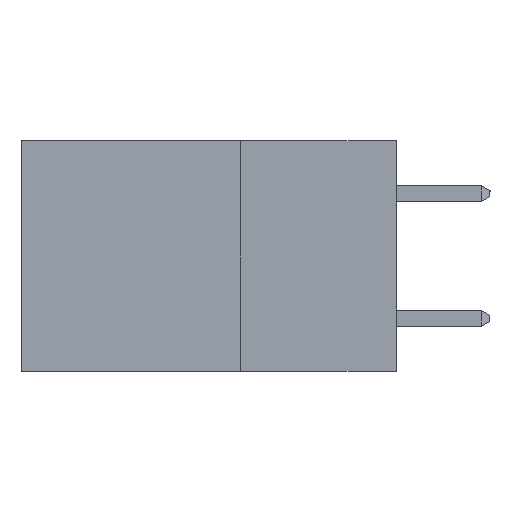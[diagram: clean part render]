
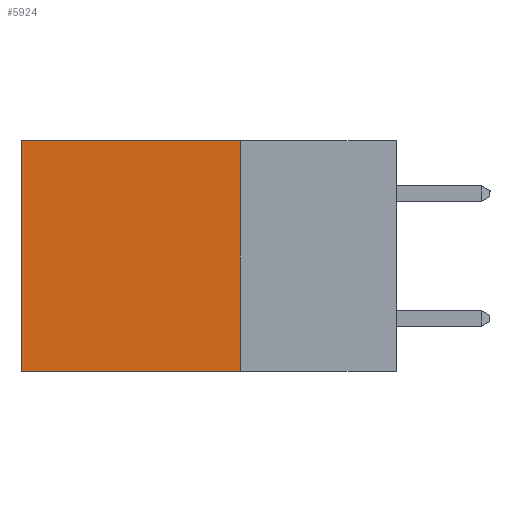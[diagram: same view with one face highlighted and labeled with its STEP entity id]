
A CAD part, left-side view. The second image highlights one B-rep face of the part: STEP entity #5924.
In plain terms, the highlighted planar face has unit normal (-1, 0, 0).
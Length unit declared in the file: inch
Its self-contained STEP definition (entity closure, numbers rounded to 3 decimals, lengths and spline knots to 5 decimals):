
#602 = FACE_OUTER_BOUND ( 'NONE', #11134, .T. ) ;
#673 = CARTESIAN_POINT ( 'NONE',  ( 0.2615, 0.25, -0.37 ) ) ;
#966 = EDGE_CURVE ( 'NONE', #3052, #10866, #13611, .T. ) ;
#971 = AXIS2_PLACEMENT_3D ( 'NONE', #13000, #1486, #2740 ) ;
#1252 = DIRECTION ( 'NONE',  ( 0., 1., 0. ) ) ;
#1486 = DIRECTION ( 'NONE',  ( 1., 0., 0. ) ) ;
#2083 = LINE ( 'NONE', #673, #9525 ) ;
#2234 = CARTESIAN_POINT ( 'NONE',  ( 0.2615, 0.6, -0.37 ) ) ;
#2464 = EDGE_CURVE ( 'NONE', #6318, #4878, #8167, .T. ) ;
#2740 = DIRECTION ( 'NONE',  ( 0., 0., -1. ) ) ;
#3030 = DIRECTION ( 'NONE',  ( 0., 1., 0. ) ) ;
#3052 = VERTEX_POINT ( 'NONE', #8642 ) ;
#3183 = CARTESIAN_POINT ( 'NONE',  ( 0.2615, 0.25, 0. ) ) ;
#3270 = DIRECTION ( 'NONE',  ( 0., 0., -1. ) ) ;
#3644 = EDGE_CURVE ( 'NONE', #6318, #3052, #11485, .T. ) ;
#4128 = ORIENTED_EDGE ( 'NONE', *, *, #966, .T. ) ;
#4236 = CARTESIAN_POINT ( 'NONE',  ( 0.2615, 0.6, -0.37 ) ) ;
#4377 = CARTESIAN_POINT ( 'NONE',  ( 0.2615, 0.25, -0.37 ) ) ;
#4671 = VECTOR ( 'NONE', #1252, 39.37008 ) ;
#4676 = EDGE_CURVE ( 'NONE', #4878, #10866, #2083, .T. ) ;
#4878 = VERTEX_POINT ( 'NONE', #4377 ) ;
#5086 = CARTESIAN_POINT ( 'NONE',  ( 0.2615, 0.25, 0. ) ) ;
#5924 = ADVANCED_FACE ( 'NONE', ( #602 ), #10529, .F. ) ;
#6318 = VERTEX_POINT ( 'NONE', #5086 ) ;
#7287 = ORIENTED_EDGE ( 'NONE', *, *, #4676, .F. ) ;
#7858 = VECTOR ( 'NONE', #3270, 39.37008 ) ;
#8167 = LINE ( 'NONE', #9521, #11370 ) ;
#8642 = CARTESIAN_POINT ( 'NONE',  ( 0.2615, 0.6, 0. ) ) ;
#9521 = CARTESIAN_POINT ( 'NONE',  ( 0.2615, 0.25, -0.37 ) ) ;
#9525 = VECTOR ( 'NONE', #3030, 39.37008 ) ;
#10529 = PLANE ( 'NONE',  #971 ) ;
#10866 = VERTEX_POINT ( 'NONE', #4236 ) ;
#11010 = ORIENTED_EDGE ( 'NONE', *, *, #2464, .F. ) ;
#11134 = EDGE_LOOP ( 'NONE', ( #4128, #7287, #11010, #12591 ) ) ;
#11370 = VECTOR ( 'NONE', #14105, 39.37008 ) ;
#11485 = LINE ( 'NONE', #3183, #4671 ) ;
#12591 = ORIENTED_EDGE ( 'NONE', *, *, #3644, .T. ) ;
#13000 = CARTESIAN_POINT ( 'NONE',  ( 0.2615, 0.25, -0.37 ) ) ;
#13611 = LINE ( 'NONE', #2234, #7858 ) ;
#14105 = DIRECTION ( 'NONE',  ( 0., 0., -1. ) ) ;
